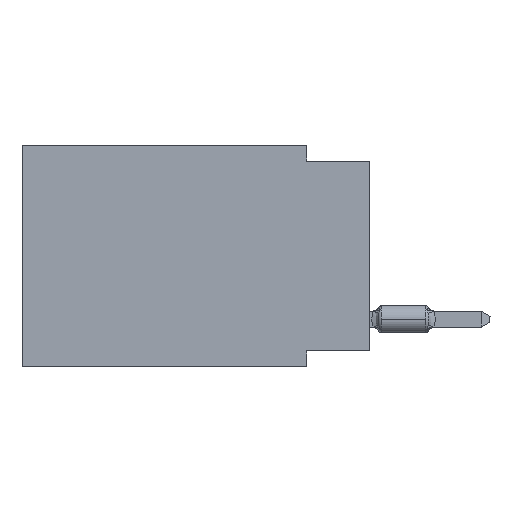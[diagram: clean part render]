
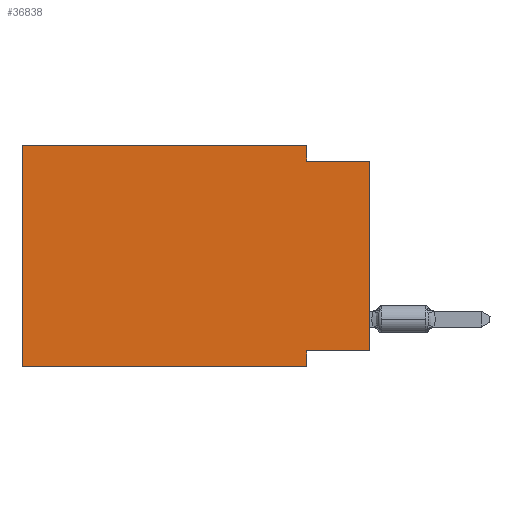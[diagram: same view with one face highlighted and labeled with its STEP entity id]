
A CAD part, left-side view. The second image highlights one B-rep face of the part: STEP entity #36838.
In plain terms, the highlighted planar face has unit normal (-1, 0, 0).
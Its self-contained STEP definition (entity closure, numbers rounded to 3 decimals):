
#391 = DIRECTION ( 'NONE',  ( 1., 0., 0. ) ) ;
#1444 = VERTEX_POINT ( 'NONE', #40706 ) ;
#1779 = LINE ( 'NONE', #53381, #72153 ) ;
#1871 = EDGE_CURVE ( 'NONE', #14014, #25381, #3244, .T. ) ;
#3244 = LINE ( 'NONE', #28002, #78505 ) ;
#6838 = EDGE_CURVE ( 'NONE', #1444, #81748, #1779, .T. ) ;
#8899 = DIRECTION ( 'NONE',  ( 0., -1., 0. ) ) ;
#9606 = VECTOR ( 'NONE', #62522, 1000. ) ;
#9613 = LINE ( 'NONE', #28916, #50770 ) ;
#10845 = CARTESIAN_POINT ( 'NONE',  ( 0., 2.54, 0. ) ) ;
#11575 = LINE ( 'NONE', #37170, #23210 ) ;
#11969 = ORIENTED_EDGE ( 'NONE', *, *, #31031, .F. ) ;
#14014 = VERTEX_POINT ( 'NONE', #82556 ) ;
#14288 = VERTEX_POINT ( 'NONE', #14987 ) ;
#14549 = CARTESIAN_POINT ( 'NONE',  ( 0., 2.54, -8.255 ) ) ;
#14987 = CARTESIAN_POINT ( 'NONE',  ( 0., 0., -8.255 ) ) ;
#18459 = FACE_OUTER_BOUND ( 'NONE', #53715, .T. ) ;
#20751 = CARTESIAN_POINT ( 'NONE',  ( 0., 2.54, -0.635 ) ) ;
#23210 = VECTOR ( 'NONE', #42636, 1000. ) ;
#25381 = VERTEX_POINT ( 'NONE', #10845 ) ;
#28002 = CARTESIAN_POINT ( 'NONE',  ( 0., 13.97, 0. ) ) ;
#28916 = CARTESIAN_POINT ( 'NONE',  ( 0., 2.54, 0. ) ) ;
#31031 = EDGE_CURVE ( 'NONE', #70810, #81748, #39857, .T. ) ;
#31867 = CARTESIAN_POINT ( 'NONE',  ( 0., 13.97, 0. ) ) ;
#32021 = AXIS2_PLACEMENT_3D ( 'NONE', #31867, #391, #51582 ) ;
#33939 = VERTEX_POINT ( 'NONE', #46435 ) ;
#36838 = ADVANCED_FACE ( 'NONE', ( #18459 ), #57854, .F. ) ;
#37170 = CARTESIAN_POINT ( 'NONE',  ( 0., 0., -0.635 ) ) ;
#37355 = VECTOR ( 'NONE', #76466, 1000. ) ;
#37680 = ORIENTED_EDGE ( 'NONE', *, *, #64429, .F. ) ;
#39857 = LINE ( 'NONE', #65422, #78286 ) ;
#40706 = CARTESIAN_POINT ( 'NONE',  ( 0., 13.97, -8.89 ) ) ;
#41089 = DIRECTION ( 'NONE',  ( 0., 0., -1. ) ) ;
#41559 = CARTESIAN_POINT ( 'NONE',  ( 0., 2.54, -8.89 ) ) ;
#42636 = DIRECTION ( 'NONE',  ( 0., -1., 0. ) ) ;
#43723 = ORIENTED_EDGE ( 'NONE', *, *, #57248, .F. ) ;
#44797 = VECTOR ( 'NONE', #65300, 1000. ) ;
#46435 = CARTESIAN_POINT ( 'NONE',  ( 0., 0., -0.635 ) ) ;
#46441 = CARTESIAN_POINT ( 'NONE',  ( 0., 0., -8.255 ) ) ;
#46898 = DIRECTION ( 'NONE',  ( 0., -1., 0. ) ) ;
#50770 = VECTOR ( 'NONE', #66676, 1000. ) ;
#51582 = DIRECTION ( 'NONE',  ( 0., 0., -1. ) ) ;
#51722 = CARTESIAN_POINT ( 'NONE',  ( 0., 13.97, 0. ) ) ;
#52755 = ORIENTED_EDGE ( 'NONE', *, *, #6838, .T. ) ;
#53381 = CARTESIAN_POINT ( 'NONE',  ( 0., 13.97, -8.89 ) ) ;
#53715 = EDGE_LOOP ( 'NONE', ( #73055, #37680, #65431, #72950, #43723, #52755, #11969, #67714 ) ) ;
#57248 = EDGE_CURVE ( 'NONE', #1444, #14014, #78114, .T. ) ;
#57752 = EDGE_CURVE ( 'NONE', #25381, #70468, #9613, .T. ) ;
#57854 = PLANE ( 'NONE',  #32021 ) ;
#62107 = CARTESIAN_POINT ( 'NONE',  ( 0., 0., 0. ) ) ;
#62522 = DIRECTION ( 'NONE',  ( 0., 0., 1. ) ) ;
#64429 = EDGE_CURVE ( 'NONE', #70468, #33939, #11575, .T. ) ;
#65300 = DIRECTION ( 'NONE',  ( 0., 1., 0. ) ) ;
#65422 = CARTESIAN_POINT ( 'NONE',  ( 0., 2.54, -8.89 ) ) ;
#65431 = ORIENTED_EDGE ( 'NONE', *, *, #57752, .F. ) ;
#65701 = EDGE_CURVE ( 'NONE', #14288, #70810, #76642, .T. ) ;
#66676 = DIRECTION ( 'NONE',  ( 0., 0., -1. ) ) ;
#67714 = ORIENTED_EDGE ( 'NONE', *, *, #65701, .F. ) ;
#69896 = EDGE_CURVE ( 'NONE', #14288, #33939, #74703, .T. ) ;
#70468 = VERTEX_POINT ( 'NONE', #20751 ) ;
#70810 = VERTEX_POINT ( 'NONE', #14549 ) ;
#72153 = VECTOR ( 'NONE', #8899, 1000. ) ;
#72950 = ORIENTED_EDGE ( 'NONE', *, *, #1871, .F. ) ;
#73055 = ORIENTED_EDGE ( 'NONE', *, *, #69896, .T. ) ;
#74703 = LINE ( 'NONE', #62107, #9606 ) ;
#76466 = DIRECTION ( 'NONE',  ( 0., 0., 1. ) ) ;
#76642 = LINE ( 'NONE', #46441, #44797 ) ;
#78114 = LINE ( 'NONE', #51722, #37355 ) ;
#78286 = VECTOR ( 'NONE', #41089, 1000. ) ;
#78505 = VECTOR ( 'NONE', #46898, 1000. ) ;
#81748 = VERTEX_POINT ( 'NONE', #41559 ) ;
#82556 = CARTESIAN_POINT ( 'NONE',  ( 0., 13.97, 0. ) ) ;
